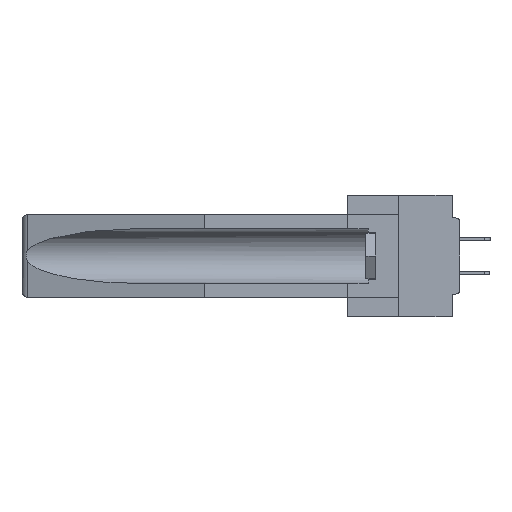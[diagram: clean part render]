
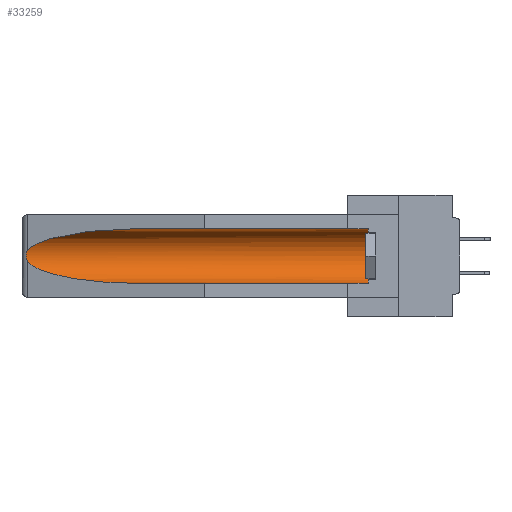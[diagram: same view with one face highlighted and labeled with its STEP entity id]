
A CAD part, left-side view. The second image highlights one B-rep face of the part: STEP entity #33259.
In plain terms, the highlighted cylindrical face has radius 2.857 mm (diameter 5.715 mm), a partial arc.
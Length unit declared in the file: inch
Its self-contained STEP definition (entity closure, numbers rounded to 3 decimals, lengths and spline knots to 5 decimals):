
#160 = VERTEX_POINT ( 'NONE', #14988 ) ;
#493 = CARTESIAN_POINT ( 'NONE',  ( 0.25451, 1.48313, -0.24835 ) ) ;
#599 = CARTESIAN_POINT ( 'NONE',  ( 0.25451, 1.48313, -0.09465 ) ) ;
#843 = CARTESIAN_POINT ( 'NONE',  ( 0.26537, 1.52718, -0.14972 ) ) ;
#1521 = CARTESIAN_POINT ( 'NONE',  ( 0.26537, 1.52718, -0.19328 ) ) ;
#1641 = B_SPLINE_CURVE_WITH_KNOTS ( 'NONE', 3,
 ( #843, #7359, #33691, #36631, #36493, #4963, #14389, #14668, #8290, #1521 ),
 .UNSPECIFIED., .F., .F.,
 ( 4, 2, 2, 2, 4 ),
 ( 0., 0.00029, 0.00058, 0.00087, 0.00117 ),
 .UNSPECIFIED. ) ;
#2644 = ORIENTED_EDGE ( 'NONE', *, *, #23916, .T. ) ;
#2962 = CARTESIAN_POINT ( 'NONE',  ( 0.155, 1.07973, -0.059 ) ) ;
#4963 = CARTESIAN_POINT ( 'NONE',  ( 0.2675, 1.53308, -0.17534 ) ) ;
#6064 = EDGE_LOOP ( 'NONE', ( #2644, #34191, #30714, #25980, #35920, #14332 ) ) ;
#6255 = AXIS2_PLACEMENT_3D ( 'NONE', #40695, #31251, #24882 ) ;
#6362 = CARTESIAN_POINT ( 'NONE',  ( 0.155, 0.126, -0.1715 ) ) ;
#7359 = CARTESIAN_POINT ( 'NONE',  ( 0.26597, 1.52961, -0.15275 ) ) ;
#7402 = CYLINDRICAL_SURFACE ( 'NONE', #6255, 0.1125 ) ;
#8290 = CARTESIAN_POINT ( 'NONE',  ( 0.26597, 1.5296, -0.19026 ) ) ;
#8667 = CARTESIAN_POINT ( 'NONE',  ( 0.155, 1.07973, -0.059 ) ) ;
#10816 =( BOUNDED_CURVE ( )  B_SPLINE_CURVE ( 3, ( #2962, #22398, #599, #26344 ),
 .UNSPECIFIED., .F., .F. ) 
 B_SPLINE_CURVE_WITH_KNOTS ( ( 4, 4 ),
 ( 4.71239, 6.08839 ),
 .UNSPECIFIED. ) 
 CURVE ( )  GEOMETRIC_REPRESENTATION_ITEM ( )  RATIONAL_B_SPLINE_CURVE ( ( 1., 0.848, 0.848, 1. ) ) 
 REPRESENTATION_ITEM ( '' )  );
#13418 = VECTOR ( 'NONE', #34228, 39.37008 ) ;
#14107 = CIRCLE ( 'NONE', #29488, 0.1125 ) ;
#14332 = ORIENTED_EDGE ( 'NONE', *, *, #20400, .T. ) ;
#14389 = CARTESIAN_POINT ( 'NONE',  ( 0.2673, 1.53269, -0.17917 ) ) ;
#14581 =( BOUNDED_CURVE ( )  B_SPLINE_CURVE ( 3, ( #25717, #493, #36252, #20429 ),
 .UNSPECIFIED., .F., .F. ) 
 B_SPLINE_CURVE_WITH_KNOTS ( ( 4, 4 ),
 ( 0.1948, 1.5708 ),
 .UNSPECIFIED. ) 
 CURVE ( )  GEOMETRIC_REPRESENTATION_ITEM ( )  RATIONAL_B_SPLINE_CURVE ( ( 1., 0.848, 0.848, 1. ) ) 
 REPRESENTATION_ITEM ( '' )  );
#14668 = CARTESIAN_POINT ( 'NONE',  ( 0.26655, 1.53094, -0.18657 ) ) ;
#14988 = CARTESIAN_POINT ( 'NONE',  ( 0.26537, 1.52718, -0.14972 ) ) ;
#17095 = EDGE_CURVE ( 'NONE', #160, #28278, #1641, .T. ) ;
#18406 = CARTESIAN_POINT ( 'NONE',  ( 0.155, 0.126, -0.059 ) ) ;
#20329 = CARTESIAN_POINT ( 'NONE',  ( 0.155, -0.30754, -0.059 ) ) ;
#20400 = EDGE_CURVE ( 'NONE', #29112, #30594, #31925, .T. ) ;
#20429 = CARTESIAN_POINT ( 'NONE',  ( 0.155, 1.07973, -0.284 ) ) ;
#21475 = CARTESIAN_POINT ( 'NONE',  ( 0.155, -0.30754, -0.284 ) ) ;
#21599 = EDGE_CURVE ( 'NONE', #28610, #33905, #27271, .T. ) ;
#21754 = DIRECTION ( 'NONE',  ( 0., -1., 0. ) ) ;
#22398 = CARTESIAN_POINT ( 'NONE',  ( 0.21114, 1.30732, -0.059 ) ) ;
#23916 = EDGE_CURVE ( 'NONE', #30594, #160, #10816, .T. ) ;
#24882 = DIRECTION ( 'NONE',  ( 0., 0., 1. ) ) ;
#25717 = CARTESIAN_POINT ( 'NONE',  ( 0.26537, 1.52718, -0.19328 ) ) ;
#25980 = ORIENTED_EDGE ( 'NONE', *, *, #21599, .F. ) ;
#26344 = CARTESIAN_POINT ( 'NONE',  ( 0.26537, 1.52718, -0.14972 ) ) ;
#27271 = LINE ( 'NONE', #21475, #13418 ) ;
#28278 = VERTEX_POINT ( 'NONE', #37822 ) ;
#28610 = VERTEX_POINT ( 'NONE', #37640 ) ;
#28782 = FACE_OUTER_BOUND ( 'NONE', #6064, .T. ) ;
#29112 = VERTEX_POINT ( 'NONE', #18406 ) ;
#29488 = AXIS2_PLACEMENT_3D ( 'NONE', #6362, #21754, #34652 ) ;
#30594 = VERTEX_POINT ( 'NONE', #8667 ) ;
#30714 = ORIENTED_EDGE ( 'NONE', *, *, #39657, .T. ) ;
#31251 = DIRECTION ( 'NONE',  ( 0., 1., 0. ) ) ;
#31399 = CARTESIAN_POINT ( 'NONE',  ( 0.155, 1.07973, -0.284 ) ) ;
#31925 = LINE ( 'NONE', #20329, #40822 ) ;
#33259 = ADVANCED_FACE ( 'NONE', ( #28782 ), #7402, .F. ) ;
#33691 = CARTESIAN_POINT ( 'NONE',  ( 0.26654, 1.53092, -0.15636 ) ) ;
#33905 = VERTEX_POINT ( 'NONE', #31399 ) ;
#34191 = ORIENTED_EDGE ( 'NONE', *, *, #17095, .T. ) ;
#34228 = DIRECTION ( 'NONE',  ( 0., 1., 0. ) ) ;
#34652 = DIRECTION ( 'NONE',  ( 0., 0., 1. ) ) ;
#35920 = ORIENTED_EDGE ( 'NONE', *, *, #38262, .T. ) ;
#36252 = CARTESIAN_POINT ( 'NONE',  ( 0.21114, 1.30732, -0.284 ) ) ;
#36286 = DIRECTION ( 'NONE',  ( 0., 1., 0. ) ) ;
#36493 = CARTESIAN_POINT ( 'NONE',  ( 0.2675, 1.53308, -0.16763 ) ) ;
#36631 = CARTESIAN_POINT ( 'NONE',  ( 0.2673, 1.5327, -0.16383 ) ) ;
#37640 = CARTESIAN_POINT ( 'NONE',  ( 0.155, 0.126, -0.284 ) ) ;
#37822 = CARTESIAN_POINT ( 'NONE',  ( 0.26537, 1.52718, -0.19328 ) ) ;
#38262 = EDGE_CURVE ( 'NONE', #28610, #29112, #14107, .T. ) ;
#39657 = EDGE_CURVE ( 'NONE', #28278, #33905, #14581, .T. ) ;
#40695 = CARTESIAN_POINT ( 'NONE',  ( 0.155, -0.30754, -0.1715 ) ) ;
#40822 = VECTOR ( 'NONE', #36286, 39.37008 ) ;
